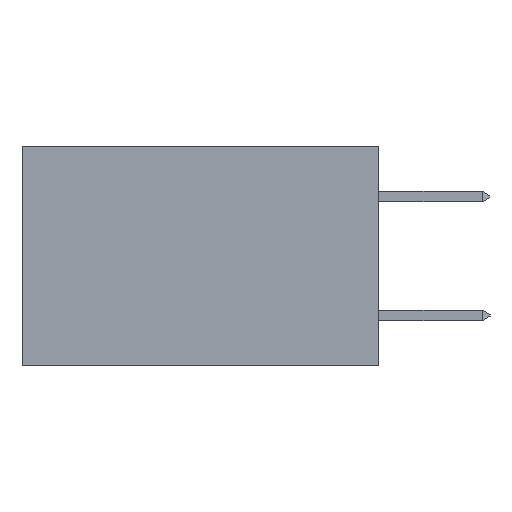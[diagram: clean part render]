
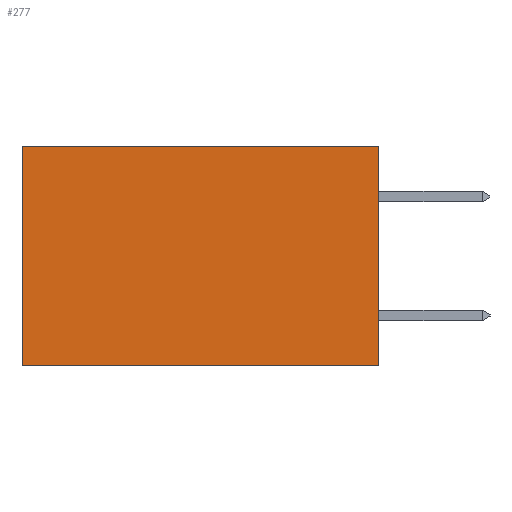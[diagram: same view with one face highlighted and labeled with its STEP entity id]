
A CAD part, left-side view. The second image highlights one B-rep face of the part: STEP entity #277.
In plain terms, the highlighted planar face has unit normal (-1, 0, 0).
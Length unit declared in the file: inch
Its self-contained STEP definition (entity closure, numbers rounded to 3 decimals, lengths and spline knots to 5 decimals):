
#277 = ADVANCED_FACE ( 'NONE', ( #11415 ), #13132, .F. ) ;
#862 = EDGE_CURVE ( 'NONE', #14929, #2304, #963, .T. ) ;
#898 = CARTESIAN_POINT ( 'NONE',  ( 0.2615, 0., 0. ) ) ;
#924 = EDGE_CURVE ( 'NONE', #8723, #14929, #15845, .T. ) ;
#963 = LINE ( 'NONE', #13778, #7847 ) ;
#1599 = ORIENTED_EDGE ( 'NONE', *, *, #862, .F. ) ;
#2054 = CARTESIAN_POINT ( 'NONE',  ( 0.2615, 0.6, 0. ) ) ;
#2304 = VERTEX_POINT ( 'NONE', #7370 ) ;
#2762 = EDGE_CURVE ( 'NONE', #11741, #2304, #14953, .T. ) ;
#3024 = VECTOR ( 'NONE', #14666, 39.37008 ) ;
#3620 = ORIENTED_EDGE ( 'NONE', *, *, #2762, .T. ) ;
#4241 = ORIENTED_EDGE ( 'NONE', *, *, #7442, .T. ) ;
#5242 = CARTESIAN_POINT ( 'NONE',  ( 0.2615, 0., -0.37 ) ) ;
#6189 = DIRECTION ( 'NONE',  ( 0., 1., 0. ) ) ;
#6501 = EDGE_LOOP ( 'NONE', ( #3620, #1599, #9975, #4241 ) ) ;
#6614 = DIRECTION ( 'NONE',  ( 0., 0., -1. ) ) ;
#6945 = CARTESIAN_POINT ( 'NONE',  ( 0.2615, 0.6, -0.37 ) ) ;
#7370 = CARTESIAN_POINT ( 'NONE',  ( 0.2615, 0.6, -0.37 ) ) ;
#7442 = EDGE_CURVE ( 'NONE', #8723, #11741, #13410, .T. ) ;
#7847 = VECTOR ( 'NONE', #6189, 39.37008 ) ;
#8723 = VERTEX_POINT ( 'NONE', #898 ) ;
#9975 = ORIENTED_EDGE ( 'NONE', *, *, #924, .F. ) ;
#11176 = AXIS2_PLACEMENT_3D ( 'NONE', #12734, #12819, #12785 ) ;
#11415 = FACE_OUTER_BOUND ( 'NONE', #6501, .T. ) ;
#11741 = VERTEX_POINT ( 'NONE', #2054 ) ;
#12021 = VECTOR ( 'NONE', #6614, 39.37008 ) ;
#12734 = CARTESIAN_POINT ( 'NONE',  ( 0.2615, 0., -0.37 ) ) ;
#12785 = DIRECTION ( 'NONE',  ( 0., 0., -1. ) ) ;
#12819 = DIRECTION ( 'NONE',  ( 1., 0., 0. ) ) ;
#13132 = PLANE ( 'NONE',  #11176 ) ;
#13410 = LINE ( 'NONE', #14958, #13739 ) ;
#13739 = VECTOR ( 'NONE', #14373, 39.37008 ) ;
#13778 = CARTESIAN_POINT ( 'NONE',  ( 0.2615, 0., -0.37 ) ) ;
#14373 = DIRECTION ( 'NONE',  ( 0., 1., 0. ) ) ;
#14666 = DIRECTION ( 'NONE',  ( 0., 0., -1. ) ) ;
#14929 = VERTEX_POINT ( 'NONE', #5242 ) ;
#14953 = LINE ( 'NONE', #6945, #12021 ) ;
#14958 = CARTESIAN_POINT ( 'NONE',  ( 0.2615, 0., 0. ) ) ;
#15123 = CARTESIAN_POINT ( 'NONE',  ( 0.2615, 0., -0.37 ) ) ;
#15845 = LINE ( 'NONE', #15123, #3024 ) ;
